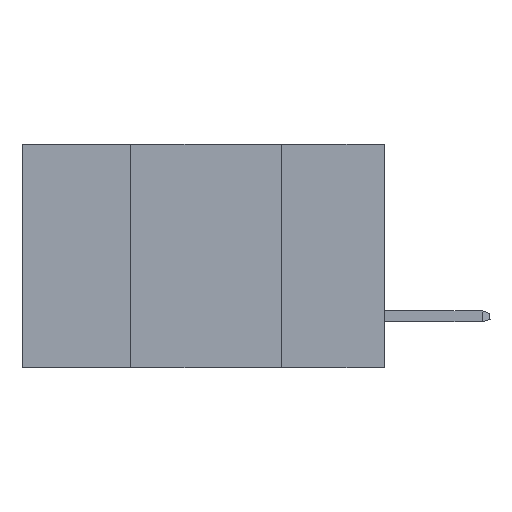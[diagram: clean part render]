
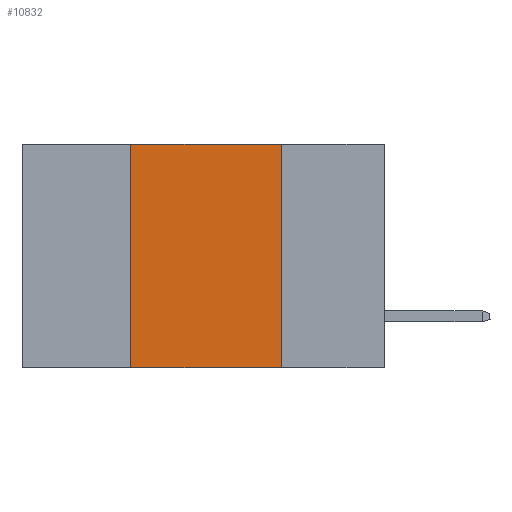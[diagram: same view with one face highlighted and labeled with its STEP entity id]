
A CAD part, left-side view. The second image highlights one B-rep face of the part: STEP entity #10832.
In plain terms, the highlighted planar face has unit normal (-1, 0, 0).
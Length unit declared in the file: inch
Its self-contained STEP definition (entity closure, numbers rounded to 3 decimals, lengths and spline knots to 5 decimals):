
#161 = CARTESIAN_POINT ( 'NONE',  ( 0., 0.42, 0. ) ) ;
#657 = EDGE_CURVE ( 'NONE', #10462, #13546, #9189, .T. ) ;
#785 = EDGE_LOOP ( 'NONE', ( #3451, #4615, #13707, #8675 ) ) ;
#814 = DIRECTION ( 'NONE',  ( 1., 0., 0. ) ) ;
#1774 = CARTESIAN_POINT ( 'NONE',  ( 0., 0.6, 0. ) ) ;
#2218 = CARTESIAN_POINT ( 'NONE',  ( 0., 0.17, 0. ) ) ;
#3106 = LINE ( 'NONE', #2218, #5029 ) ;
#3451 = ORIENTED_EDGE ( 'NONE', *, *, #8663, .F. ) ;
#4602 = VECTOR ( 'NONE', #8472, 39.37008 ) ;
#4615 = ORIENTED_EDGE ( 'NONE', *, *, #6106, .F. ) ;
#4822 = CARTESIAN_POINT ( 'NONE',  ( 0., 0.17, 0. ) ) ;
#5029 = VECTOR ( 'NONE', #6643, 39.37008 ) ;
#5256 = DIRECTION ( 'NONE',  ( 0., -1., 0. ) ) ;
#6106 = EDGE_CURVE ( 'NONE', #13546, #8752, #9239, .T. ) ;
#6203 = PLANE ( 'NONE',  #6787 ) ;
#6570 = VECTOR ( 'NONE', #5256, 39.37008 ) ;
#6612 = DIRECTION ( 'NONE',  ( 0., 0., 1. ) ) ;
#6643 = DIRECTION ( 'NONE',  ( 0., 0., -1. ) ) ;
#6787 = AXIS2_PLACEMENT_3D ( 'NONE', #1774, #814, #8411 ) ;
#6927 = FACE_OUTER_BOUND ( 'NONE', #785, .T. ) ;
#7181 = CARTESIAN_POINT ( 'NONE',  ( 0., 0.6, 0. ) ) ;
#7249 = CARTESIAN_POINT ( 'NONE',  ( 0., 0.42, 0. ) ) ;
#7775 = CARTESIAN_POINT ( 'NONE',  ( 0., 0.17, -0.37 ) ) ;
#8052 = VERTEX_POINT ( 'NONE', #7775 ) ;
#8411 = DIRECTION ( 'NONE',  ( 0., 0., -1. ) ) ;
#8472 = DIRECTION ( 'NONE',  ( 0., -1., 0. ) ) ;
#8663 = EDGE_CURVE ( 'NONE', #8752, #8052, #3106, .T. ) ;
#8675 = ORIENTED_EDGE ( 'NONE', *, *, #10169, .T. ) ;
#8723 = CARTESIAN_POINT ( 'NONE',  ( 0., 0.6, -0.37 ) ) ;
#8752 = VERTEX_POINT ( 'NONE', #4822 ) ;
#9189 = LINE ( 'NONE', #161, #9874 ) ;
#9239 = LINE ( 'NONE', #7181, #4602 ) ;
#9874 = VECTOR ( 'NONE', #6612, 39.37008 ) ;
#10169 = EDGE_CURVE ( 'NONE', #10462, #8052, #10689, .T. ) ;
#10462 = VERTEX_POINT ( 'NONE', #12276 ) ;
#10689 = LINE ( 'NONE', #8723, #6570 ) ;
#10832 = ADVANCED_FACE ( 'NONE', ( #6927 ), #6203, .F. ) ;
#12276 = CARTESIAN_POINT ( 'NONE',  ( 0., 0.42, -0.37 ) ) ;
#13546 = VERTEX_POINT ( 'NONE', #7249 ) ;
#13707 = ORIENTED_EDGE ( 'NONE', *, *, #657, .F. ) ;
